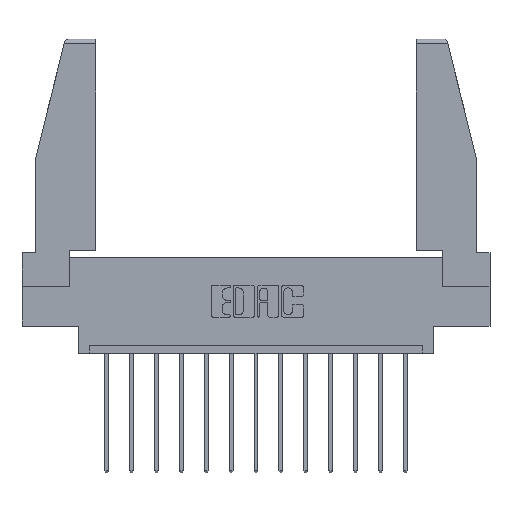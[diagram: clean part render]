
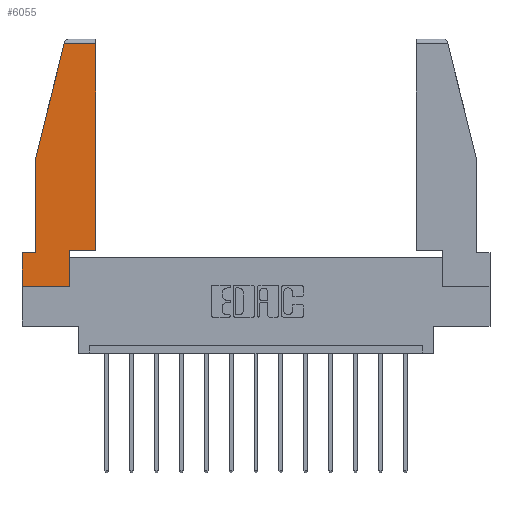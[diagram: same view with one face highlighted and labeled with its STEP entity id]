
A CAD part, top view. The second image highlights one B-rep face of the part: STEP entity #6055.
In plain terms, the highlighted planar face has unit normal (0, 0, 1).
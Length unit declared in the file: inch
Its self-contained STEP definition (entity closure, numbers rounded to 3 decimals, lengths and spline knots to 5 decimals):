
#1411 = ORIENTED_EDGE ( 'NONE', *, *, #6224, .T. ) ;
#1855 = VERTEX_POINT ( 'NONE', #13710 ) ;
#1934 = VECTOR ( 'NONE', #10896, 39.37008 ) ;
#2368 = LINE ( 'NONE', #8161, #11833 ) ;
#2876 = DIRECTION ( 'NONE',  ( 0., -1., 0. ) ) ;
#2936 = ORIENTED_EDGE ( 'NONE', *, *, #5734, .T. ) ;
#3154 = LINE ( 'NONE', #4244, #6837 ) ;
#3221 = LINE ( 'NONE', #4351, #9393 ) ;
#3287 = VERTEX_POINT ( 'NONE', #12844 ) ;
#3563 = EDGE_CURVE ( 'NONE', #7042, #5660, #14396, .T. ) ;
#3682 = EDGE_CURVE ( 'NONE', #3287, #7042, #8190, .T. ) ;
#3686 = CARTESIAN_POINT ( 'NONE',  ( 0.461, 0.223, 0. ) ) ;
#4151 = CARTESIAN_POINT ( 'NONE',  ( 0., 0.21, 0. ) ) ;
#4244 = CARTESIAN_POINT ( 'NONE',  ( 0., 1.52, 0. ) ) ;
#4351 = CARTESIAN_POINT ( 'NONE',  ( 0.297, 0.223, 0. ) ) ;
#4516 = CARTESIAN_POINT ( 'NONE',  ( 0., 0., 0. ) ) ;
#4788 = AXIS2_PLACEMENT_3D ( 'NONE', #6611, #15293, #10432 ) ;
#4903 = FACE_OUTER_BOUND ( 'NONE', #8739, .T. ) ;
#5036 = ORIENTED_EDGE ( 'NONE', *, *, #14065, .T. ) ;
#5203 = ORIENTED_EDGE ( 'NONE', *, *, #12366, .T. ) ;
#5500 = ORIENTED_EDGE ( 'NONE', *, *, #3563, .T. ) ;
#5551 = EDGE_CURVE ( 'NONE', #11554, #12574, #3154, .T. ) ;
#5660 = VERTEX_POINT ( 'NONE', #4516 ) ;
#5734 = EDGE_CURVE ( 'NONE', #5660, #15584, #6457, .T. ) ;
#6055 = ADVANCED_FACE ( 'NONE', ( #4903 ), #11661, .T. ) ;
#6198 = CARTESIAN_POINT ( 'NONE',  ( 0., 0.21, 0. ) ) ;
#6224 = EDGE_CURVE ( 'NONE', #8722, #11554, #2368, .T. ) ;
#6329 = VECTOR ( 'NONE', #15886, 39.37008 ) ;
#6457 = LINE ( 'NONE', #11839, #15915 ) ;
#6611 = CARTESIAN_POINT ( 'NONE',  ( 0., 0., 0. ) ) ;
#6837 = VECTOR ( 'NONE', #12733, 39.37008 ) ;
#7038 = DIRECTION ( 'NONE',  ( -1., 0., 0. ) ) ;
#7042 = VERTEX_POINT ( 'NONE', #4151 ) ;
#7123 = VECTOR ( 'NONE', #2876, 39.37008 ) ;
#8019 = CARTESIAN_POINT ( 'NONE',  ( 0.2636, 1.52, 0. ) ) ;
#8161 = CARTESIAN_POINT ( 'NONE',  ( 0.461, 0.223, 0. ) ) ;
#8190 = LINE ( 'NONE', #6198, #9915 ) ;
#8311 = CARTESIAN_POINT ( 'NONE',  ( 0.297, 0., 0. ) ) ;
#8722 = VERTEX_POINT ( 'NONE', #3686 ) ;
#8739 = EDGE_LOOP ( 'NONE', ( #1411, #11511, #5036, #13597, #10990, #5500, #2936, #5203, #12646 ) ) ;
#8837 = CARTESIAN_POINT ( 'NONE',  ( 0., 0.21, 0. ) ) ;
#9150 = CARTESIAN_POINT ( 'NONE',  ( 0.461, 1.52, 0. ) ) ;
#9276 = DIRECTION ( 'NONE',  ( 0., 1., 0. ) ) ;
#9393 = VECTOR ( 'NONE', #11943, 39.37008 ) ;
#9915 = VECTOR ( 'NONE', #7038, 39.37008 ) ;
#10080 = DIRECTION ( 'NONE',  ( 0., -1., 0. ) ) ;
#10421 = LINE ( 'NONE', #11614, #7123 ) ;
#10432 = DIRECTION ( 'NONE',  ( 1., 0., 0. ) ) ;
#10493 = DIRECTION ( 'NONE',  ( 1., 0., 0. ) ) ;
#10891 = VECTOR ( 'NONE', #10080, 39.37008 ) ;
#10896 = DIRECTION ( 'NONE',  ( 0., 1., 0. ) ) ;
#10928 = VERTEX_POINT ( 'NONE', #11550 ) ;
#10990 = ORIENTED_EDGE ( 'NONE', *, *, #3682, .T. ) ;
#11511 = ORIENTED_EDGE ( 'NONE', *, *, #5551, .T. ) ;
#11521 = LINE ( 'NONE', #15349, #6329 ) ;
#11550 = CARTESIAN_POINT ( 'NONE',  ( 0.297, 0.223, 0. ) ) ;
#11554 = VERTEX_POINT ( 'NONE', #9150 ) ;
#11614 = CARTESIAN_POINT ( 'NONE',  ( 0.086, 0.8, 0. ) ) ;
#11661 = PLANE ( 'NONE',  #4788 ) ;
#11833 = VECTOR ( 'NONE', #9276, 39.37008 ) ;
#11839 = CARTESIAN_POINT ( 'NONE',  ( 0., 0., 0. ) ) ;
#11943 = DIRECTION ( 'NONE',  ( 1., 0., 0. ) ) ;
#12366 = EDGE_CURVE ( 'NONE', #15584, #10928, #13924, .T. ) ;
#12574 = VERTEX_POINT ( 'NONE', #8019 ) ;
#12646 = ORIENTED_EDGE ( 'NONE', *, *, #13834, .T. ) ;
#12726 = EDGE_CURVE ( 'NONE', #1855, #3287, #10421, .T. ) ;
#12733 = DIRECTION ( 'NONE',  ( -1., 0., 0. ) ) ;
#12844 = CARTESIAN_POINT ( 'NONE',  ( 0.086, 0.21, 0. ) ) ;
#13597 = ORIENTED_EDGE ( 'NONE', *, *, #12726, .T. ) ;
#13710 = CARTESIAN_POINT ( 'NONE',  ( 0.086, 0.8, 0. ) ) ;
#13834 = EDGE_CURVE ( 'NONE', #10928, #8722, #3221, .T. ) ;
#13924 = LINE ( 'NONE', #15857, #1934 ) ;
#14065 = EDGE_CURVE ( 'NONE', #12574, #1855, #11521, .T. ) ;
#14396 = LINE ( 'NONE', #8837, #10891 ) ;
#15293 = DIRECTION ( 'NONE',  ( 0., 0., 1. ) ) ;
#15349 = CARTESIAN_POINT ( 'NONE',  ( 0.271, 1.55, 0. ) ) ;
#15584 = VERTEX_POINT ( 'NONE', #8311 ) ;
#15857 = CARTESIAN_POINT ( 'NONE',  ( 0.297, 0., 0. ) ) ;
#15886 = DIRECTION ( 'NONE',  ( -0.239, -0.971, 0. ) ) ;
#15915 = VECTOR ( 'NONE', #10493, 39.37008 ) ;
